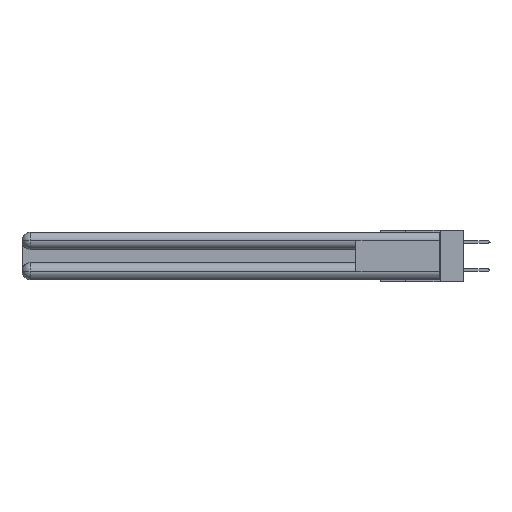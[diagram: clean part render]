
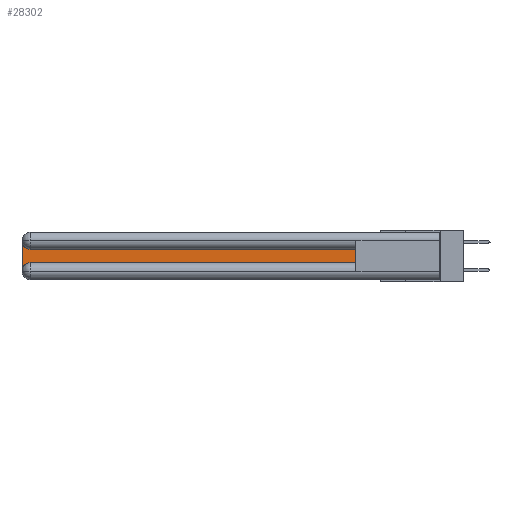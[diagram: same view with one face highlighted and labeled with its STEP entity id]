
A CAD part, left-side view. The second image highlights one B-rep face of the part: STEP entity #28302.
In plain terms, the highlighted planar face has unit normal (-1, 0, 0).
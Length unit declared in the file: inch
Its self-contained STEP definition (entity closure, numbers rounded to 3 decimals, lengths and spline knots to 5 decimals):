
#1140 = VERTEX_POINT ( 'NONE', #4041 ) ;
#1176 = LINE ( 'NONE', #23026, #21673 ) ;
#1594 = VECTOR ( 'NONE', #14695, 39.37008 ) ;
#3200 = DIRECTION ( 'NONE',  ( 1., 0., 0. ) ) ;
#3313 = PLANE ( 'NONE',  #27278 ) ;
#3623 = AXIS2_PLACEMENT_3D ( 'NONE', #7566, #10000, #19386 ) ;
#3735 = CARTESIAN_POINT ( 'NONE',  ( 0.075, 0.6, -0.2175 ) ) ;
#3842 = DIRECTION ( 'NONE',  ( 0., 0., -1. ) ) ;
#4041 = CARTESIAN_POINT ( 'NONE',  ( 0.075, 0.6, -0.2175 ) ) ;
#5298 = ORIENTED_EDGE ( 'NONE', *, *, #22757, .T. ) ;
#6029 = LINE ( 'NONE', #25518, #18454 ) ;
#6635 = CIRCLE ( 'NONE', #3623, 0.06 ) ;
#6770 = ORIENTED_EDGE ( 'NONE', *, *, #10197, .T. ) ;
#7566 = CARTESIAN_POINT ( 'NONE',  ( 0.075, 2.94, -0.2775 ) ) ;
#7960 = VERTEX_POINT ( 'NONE', #19602 ) ;
#8994 = ORIENTED_EDGE ( 'NONE', *, *, #12857, .T. ) ;
#9504 = EDGE_CURVE ( 'NONE', #18712, #7960, #1176, .T. ) ;
#10000 = DIRECTION ( 'NONE',  ( 1., 0., 0. ) ) ;
#10197 = EDGE_CURVE ( 'NONE', #7960, #21074, #6635, .T. ) ;
#10369 = EDGE_LOOP ( 'NONE', ( #26217, #29378, #17895, #6770, #5298, #8994 ) ) ;
#10770 = CARTESIAN_POINT ( 'NONE',  ( 0.075, 2.94, -0.0625 ) ) ;
#11506 = DIRECTION ( 'NONE',  ( 0., 1., 0. ) ) ;
#12496 = VERTEX_POINT ( 'NONE', #21866 ) ;
#12857 = EDGE_CURVE ( 'NONE', #1140, #13618, #25445, .T. ) ;
#13618 = VERTEX_POINT ( 'NONE', #25076 ) ;
#14558 = CARTESIAN_POINT ( 'NONE',  ( 0.075, 3., -0.0625 ) ) ;
#14695 = DIRECTION ( 'NONE',  ( 0., 0., 1. ) ) ;
#14947 = CARTESIAN_POINT ( 'NONE',  ( 0.075, 2.94, -0.2175 ) ) ;
#17189 = FACE_OUTER_BOUND ( 'NONE', #10369, .T. ) ;
#17262 = CARTESIAN_POINT ( 'NONE',  ( 0.075, 0.6, -0.2175 ) ) ;
#17895 = ORIENTED_EDGE ( 'NONE', *, *, #9504, .T. ) ;
#18454 = VECTOR ( 'NONE', #11506, 39.37008 ) ;
#18712 = VERTEX_POINT ( 'NONE', #14558 ) ;
#18816 = VECTOR ( 'NONE', #22441, 39.37008 ) ;
#19248 = DIRECTION ( 'NONE',  ( 0., 0., -1. ) ) ;
#19386 = DIRECTION ( 'NONE',  ( 0., 0., -1. ) ) ;
#19602 = CARTESIAN_POINT ( 'NONE',  ( 0.075, 3., -0.2775 ) ) ;
#20659 = LINE ( 'NONE', #3735, #18816 ) ;
#20848 = EDGE_CURVE ( 'NONE', #12496, #18712, #27757, .T. ) ;
#21074 = VERTEX_POINT ( 'NONE', #14947 ) ;
#21673 = VECTOR ( 'NONE', #27749, 39.37008 ) ;
#21866 = CARTESIAN_POINT ( 'NONE',  ( 0.075, 2.94, -0.1225 ) ) ;
#22441 = DIRECTION ( 'NONE',  ( 0., -1., 0. ) ) ;
#22757 = EDGE_CURVE ( 'NONE', #21074, #1140, #20659, .T. ) ;
#23026 = CARTESIAN_POINT ( 'NONE',  ( 0.075, 3., -0.2175 ) ) ;
#24918 = DIRECTION ( 'NONE',  ( 1., 0., 0. ) ) ;
#25076 = CARTESIAN_POINT ( 'NONE',  ( 0.075, 0.6, -0.1225 ) ) ;
#25445 = LINE ( 'NONE', #17262, #1594 ) ;
#25518 = CARTESIAN_POINT ( 'NONE',  ( 0.075, 0.6, -0.1225 ) ) ;
#25852 = EDGE_CURVE ( 'NONE', #13618, #12496, #6029, .T. ) ;
#26217 = ORIENTED_EDGE ( 'NONE', *, *, #25852, .T. ) ;
#26567 = CARTESIAN_POINT ( 'NONE',  ( 0.075, 3., -0.1225 ) ) ;
#27278 = AXIS2_PLACEMENT_3D ( 'NONE', #26567, #3200, #19248 ) ;
#27749 = DIRECTION ( 'NONE',  ( 0., 0., -1. ) ) ;
#27757 = CIRCLE ( 'NONE', #30070, 0.06 ) ;
#28302 = ADVANCED_FACE ( 'NONE', ( #17189 ), #3313, .F. ) ;
#29378 = ORIENTED_EDGE ( 'NONE', *, *, #20848, .T. ) ;
#30070 = AXIS2_PLACEMENT_3D ( 'NONE', #10770, #24918, #3842 ) ;
